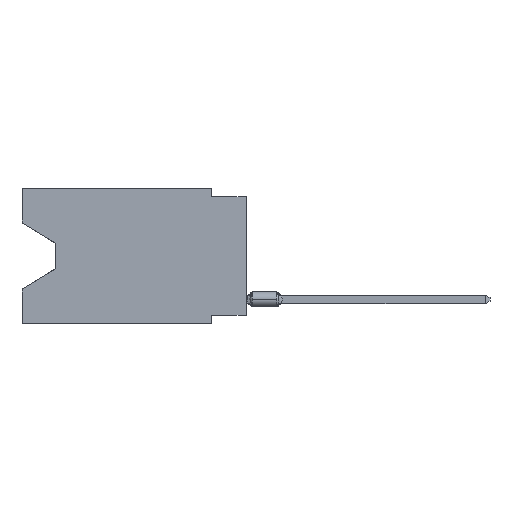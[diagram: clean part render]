
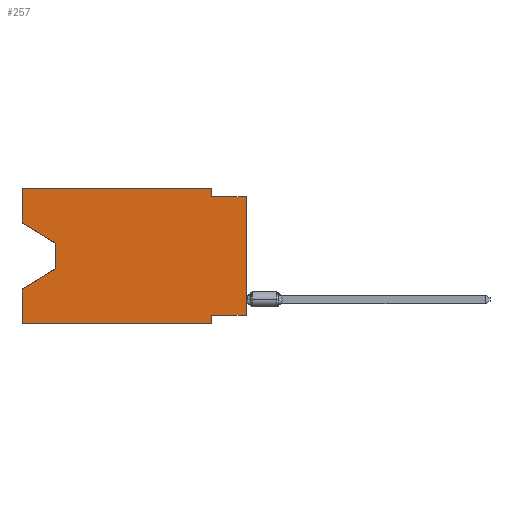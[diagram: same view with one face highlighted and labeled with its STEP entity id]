
A CAD part, left-side view. The second image highlights one B-rep face of the part: STEP entity #257.
In plain terms, the highlighted planar face has unit normal (-1, 0, 0).
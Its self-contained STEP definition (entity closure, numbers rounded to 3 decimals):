
#257 = ADVANCED_FACE ( 'NONE', ( #4552 ), #11383, .F. ) ;
#1266 = DIRECTION ( 'NONE',  ( 0., -1., 0. ) ) ;
#1404 = EDGE_CURVE ( 'NONE', #4397, #10945, #2729, .T. ) ;
#1703 = DIRECTION ( 'NONE',  ( 0., 0., -1. ) ) ;
#2448 = CARTESIAN_POINT ( 'NONE',  ( 0., 16.383, 0. ) ) ;
#2628 = DIRECTION ( 'NONE',  ( 1., 0., 0. ) ) ;
#2729 = LINE ( 'NONE', #2448, #12811 ) ;
#2957 = ORIENTED_EDGE ( 'NONE', *, *, #20537, .T. ) ;
#3133 = VECTOR ( 'NONE', #22535, 1000. ) ;
#3372 = VERTEX_POINT ( 'NONE', #17154 ) ;
#3424 = CARTESIAN_POINT ( 'NONE',  ( 0., 0., 0. ) ) ;
#3945 = CARTESIAN_POINT ( 'NONE',  ( 0., 0., -0.635 ) ) ;
#4397 = VERTEX_POINT ( 'NONE', #8173 ) ;
#4552 = FACE_OUTER_BOUND ( 'NONE', #24604, .T. ) ;
#5493 = VERTEX_POINT ( 'NONE', #5675 ) ;
#5675 = CARTESIAN_POINT ( 'NONE',  ( 0., 2.54, -0.635 ) ) ;
#5875 = VECTOR ( 'NONE', #19257, 1000. ) ;
#5948 = DIRECTION ( 'NONE',  ( 0., -0.855, -0.519 ) ) ;
#6016 = VECTOR ( 'NONE', #22776, 1000. ) ;
#6625 = CARTESIAN_POINT ( 'NONE',  ( 0., 0., -0.635 ) ) ;
#6626 = CARTESIAN_POINT ( 'NONE',  ( 0., 13.97, -5.893 ) ) ;
#6796 = VECTOR ( 'NONE', #1266, 1000. ) ;
#7379 = CARTESIAN_POINT ( 'NONE',  ( 0., 16.383, 0. ) ) ;
#7912 = LINE ( 'NONE', #21254, #6796 ) ;
#8173 = CARTESIAN_POINT ( 'NONE',  ( 0., 16.383, -9.906 ) ) ;
#8538 = VECTOR ( 'NONE', #23210, 1000. ) ;
#9704 = CARTESIAN_POINT ( 'NONE',  ( 0., 2.54, -9.271 ) ) ;
#10172 = EDGE_CURVE ( 'NONE', #3372, #5493, #22286, .T. ) ;
#10589 = ORIENTED_EDGE ( 'NONE', *, *, #26312, .F. ) ;
#10632 = VECTOR ( 'NONE', #5948, 1000. ) ;
#10688 = EDGE_CURVE ( 'NONE', #13271, #18351, #22690, .T. ) ;
#10894 = CARTESIAN_POINT ( 'NONE',  ( 0., 2.54, 0. ) ) ;
#10945 = VERTEX_POINT ( 'NONE', #17630 ) ;
#11061 = LINE ( 'NONE', #6626, #26124 ) ;
#11191 = VERTEX_POINT ( 'NONE', #7379 ) ;
#11383 = PLANE ( 'NONE',  #17471 ) ;
#11539 = EDGE_CURVE ( 'NONE', #14339, #11191, #19308, .T. ) ;
#11660 = VECTOR ( 'NONE', #25651, 1000. ) ;
#11781 = VERTEX_POINT ( 'NONE', #22836 ) ;
#11966 = LINE ( 'NONE', #12108, #8538 ) ;
#12108 = CARTESIAN_POINT ( 'NONE',  ( 0., 2.54, -9.906 ) ) ;
#12811 = VECTOR ( 'NONE', #22863, 1000. ) ;
#12923 = LINE ( 'NONE', #21936, #10632 ) ;
#13271 = VERTEX_POINT ( 'NONE', #16360 ) ;
#13342 = VERTEX_POINT ( 'NONE', #20369 ) ;
#14155 = LINE ( 'NONE', #25503, #21294 ) ;
#14339 = VERTEX_POINT ( 'NONE', #17606 ) ;
#14612 = EDGE_CURVE ( 'NONE', #18351, #11781, #11966, .T. ) ;
#14740 = DIRECTION ( 'NONE',  ( 0., 0., -1. ) ) ;
#15687 = CARTESIAN_POINT ( 'NONE',  ( 0., 16.383, 0. ) ) ;
#15812 = CARTESIAN_POINT ( 'NONE',  ( 0., 13.97, -4.013 ) ) ;
#15843 = ORIENTED_EDGE ( 'NONE', *, *, #11539, .F. ) ;
#15973 = DIRECTION ( 'NONE',  ( 0., 0., -1. ) ) ;
#16042 = EDGE_CURVE ( 'NONE', #13342, #10945, #11061, .T. ) ;
#16115 = ORIENTED_EDGE ( 'NONE', *, *, #10688, .F. ) ;
#16360 = CARTESIAN_POINT ( 'NONE',  ( 0., 0., -9.271 ) ) ;
#17154 = CARTESIAN_POINT ( 'NONE',  ( 0., 2.54, 0. ) ) ;
#17471 = AXIS2_PLACEMENT_3D ( 'NONE', #15687, #2628, #15973 ) ;
#17606 = CARTESIAN_POINT ( 'NONE',  ( 0., 16.383, -2.546 ) ) ;
#17630 = CARTESIAN_POINT ( 'NONE',  ( 0., 16.383, -7.36 ) ) ;
#17718 = DIRECTION ( 'NONE',  ( 0., -1., 0. ) ) ;
#17732 = ORIENTED_EDGE ( 'NONE', *, *, #16042, .T. ) ;
#17830 = EDGE_CURVE ( 'NONE', #14339, #27778, #12923, .T. ) ;
#17899 = LINE ( 'NONE', #22913, #6016 ) ;
#18137 = ORIENTED_EDGE ( 'NONE', *, *, #29005, .T. ) ;
#18241 = ORIENTED_EDGE ( 'NONE', *, *, #17830, .T. ) ;
#18351 = VERTEX_POINT ( 'NONE', #9704 ) ;
#19257 = DIRECTION ( 'NONE',  ( 0., 0., 1. ) ) ;
#19308 = LINE ( 'NONE', #28163, #11660 ) ;
#20369 = CARTESIAN_POINT ( 'NONE',  ( 0., 13.97, -5.893 ) ) ;
#20537 = EDGE_CURVE ( 'NONE', #4397, #11781, #17899, .T. ) ;
#20606 = CARTESIAN_POINT ( 'NONE',  ( 0., 0., -9.271 ) ) ;
#21254 = CARTESIAN_POINT ( 'NONE',  ( 0., 16.383, 0. ) ) ;
#21294 = VECTOR ( 'NONE', #14740, 1000. ) ;
#21890 = ORIENTED_EDGE ( 'NONE', *, *, #14612, .F. ) ;
#21936 = CARTESIAN_POINT ( 'NONE',  ( 0., 16.383, -2.546 ) ) ;
#22004 = LINE ( 'NONE', #3945, #27509 ) ;
#22100 = VERTEX_POINT ( 'NONE', #6625 ) ;
#22286 = LINE ( 'NONE', #10894, #27665 ) ;
#22433 = ORIENTED_EDGE ( 'NONE', *, *, #10172, .F. ) ;
#22535 = DIRECTION ( 'NONE',  ( 0., 1., 0. ) ) ;
#22690 = LINE ( 'NONE', #20606, #3133 ) ;
#22776 = DIRECTION ( 'NONE',  ( 0., -1., 0. ) ) ;
#22836 = CARTESIAN_POINT ( 'NONE',  ( 0., 2.54, -9.906 ) ) ;
#22863 = DIRECTION ( 'NONE',  ( 0., 0., 1. ) ) ;
#22913 = CARTESIAN_POINT ( 'NONE',  ( 0., 16.383, -9.906 ) ) ;
#23210 = DIRECTION ( 'NONE',  ( 0., 0., -1. ) ) ;
#24244 = EDGE_CURVE ( 'NONE', #27778, #13342, #14155, .T. ) ;
#24604 = EDGE_LOOP ( 'NONE', ( #18241, #27033, #17732, #25721, #2957, #21890, #16115, #18137, #10589, #22433, #25473, #15843 ) ) ;
#25473 = ORIENTED_EDGE ( 'NONE', *, *, #28034, .F. ) ;
#25503 = CARTESIAN_POINT ( 'NONE',  ( 0., 13.97, -4.013 ) ) ;
#25651 = DIRECTION ( 'NONE',  ( 0., 0., 1. ) ) ;
#25721 = ORIENTED_EDGE ( 'NONE', *, *, #1404, .F. ) ;
#26124 = VECTOR ( 'NONE', #26718, 1000. ) ;
#26312 = EDGE_CURVE ( 'NONE', #5493, #22100, #22004, .T. ) ;
#26718 = DIRECTION ( 'NONE',  ( 0., 0.855, -0.519 ) ) ;
#27033 = ORIENTED_EDGE ( 'NONE', *, *, #24244, .T. ) ;
#27509 = VECTOR ( 'NONE', #17718, 1000. ) ;
#27665 = VECTOR ( 'NONE', #1703, 1000. ) ;
#27778 = VERTEX_POINT ( 'NONE', #15812 ) ;
#28034 = EDGE_CURVE ( 'NONE', #11191, #3372, #7912, .T. ) ;
#28163 = CARTESIAN_POINT ( 'NONE',  ( 0., 16.383, 0. ) ) ;
#28263 = LINE ( 'NONE', #3424, #5875 ) ;
#29005 = EDGE_CURVE ( 'NONE', #13271, #22100, #28263, .T. ) ;
